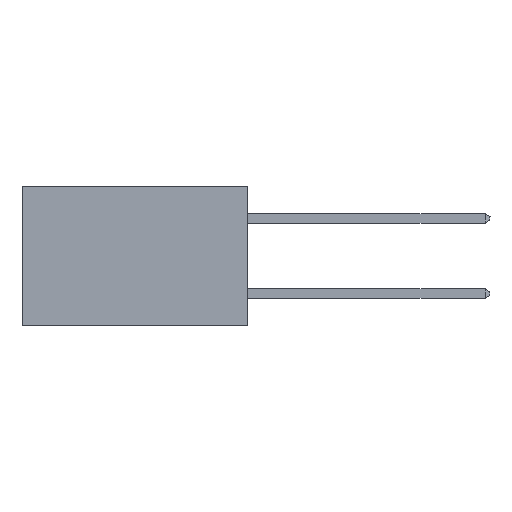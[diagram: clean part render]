
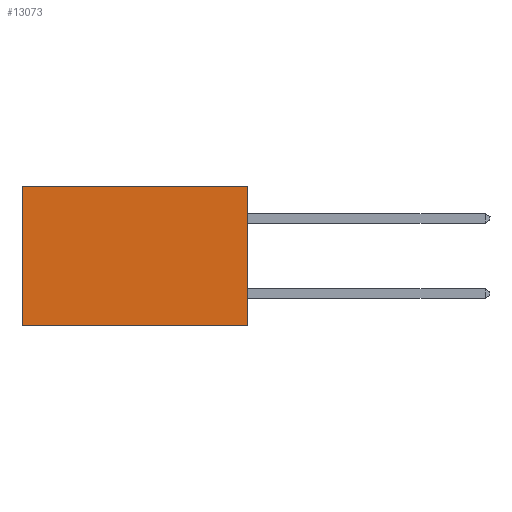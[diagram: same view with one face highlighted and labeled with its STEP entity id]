
A CAD part, left-side view. The second image highlights one B-rep face of the part: STEP entity #13073.
In plain terms, the highlighted planar face has unit normal (-1, 0, 0).
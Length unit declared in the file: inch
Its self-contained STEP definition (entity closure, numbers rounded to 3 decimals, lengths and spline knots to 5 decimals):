
#404 = CARTESIAN_POINT ( 'NONE',  ( 0.2615, 0.6, -0.37 ) ) ;
#422 = CARTESIAN_POINT ( 'NONE',  ( 0.2615, 0.6, 0. ) ) ;
#670 = CARTESIAN_POINT ( 'NONE',  ( 0.2615, 0.6, -0.37 ) ) ;
#1036 = FACE_OUTER_BOUND ( 'NONE', #8009, .T. ) ;
#2550 = VERTEX_POINT ( 'NONE', #13276 ) ;
#3620 = DIRECTION ( 'NONE',  ( 0., 0., -1. ) ) ;
#3653 = VECTOR ( 'NONE', #6985, 39.37008 ) ;
#4082 = VERTEX_POINT ( 'NONE', #670 ) ;
#4571 = ORIENTED_EDGE ( 'NONE', *, *, #7743, .T. ) ;
#4793 = CARTESIAN_POINT ( 'NONE',  ( 0.2615, 0., -0.37 ) ) ;
#4908 = VECTOR ( 'NONE', #5227, 39.37008 ) ;
#5067 = LINE ( 'NONE', #404, #15256 ) ;
#5227 = DIRECTION ( 'NONE',  ( 0., 1., 0. ) ) ;
#5365 = ORIENTED_EDGE ( 'NONE', *, *, #10840, .F. ) ;
#5797 = DIRECTION ( 'NONE',  ( 1., 0., 0. ) ) ;
#5877 = LINE ( 'NONE', #12953, #3653 ) ;
#5997 = VERTEX_POINT ( 'NONE', #15090 ) ;
#6898 = ORIENTED_EDGE ( 'NONE', *, *, #14724, .T. ) ;
#6985 = DIRECTION ( 'NONE',  ( 0., 0., -1. ) ) ;
#7135 = DIRECTION ( 'NONE',  ( 0., 1., 0. ) ) ;
#7436 = VERTEX_POINT ( 'NONE', #422 ) ;
#7646 = VECTOR ( 'NONE', #7135, 39.37008 ) ;
#7743 = EDGE_CURVE ( 'NONE', #5997, #7436, #13624, .T. ) ;
#8009 = EDGE_LOOP ( 'NONE', ( #6898, #5365, #11584, #4571 ) ) ;
#8851 = DIRECTION ( 'NONE',  ( 0., 0., -1. ) ) ;
#10460 = PLANE ( 'NONE',  #13962 ) ;
#10746 = EDGE_CURVE ( 'NONE', #5997, #2550, #5877, .T. ) ;
#10840 = EDGE_CURVE ( 'NONE', #2550, #4082, #14362, .T. ) ;
#11584 = ORIENTED_EDGE ( 'NONE', *, *, #10746, .F. ) ;
#12953 = CARTESIAN_POINT ( 'NONE',  ( 0.2615, 0., -0.37 ) ) ;
#13073 = ADVANCED_FACE ( 'NONE', ( #1036 ), #10460, .F. ) ;
#13187 = CARTESIAN_POINT ( 'NONE',  ( 0.2615, 0., -0.37 ) ) ;
#13276 = CARTESIAN_POINT ( 'NONE',  ( 0.2615, 0., -0.37 ) ) ;
#13624 = LINE ( 'NONE', #14805, #4908 ) ;
#13962 = AXIS2_PLACEMENT_3D ( 'NONE', #4793, #5797, #3620 ) ;
#14362 = LINE ( 'NONE', #13187, #7646 ) ;
#14724 = EDGE_CURVE ( 'NONE', #7436, #4082, #5067, .T. ) ;
#14805 = CARTESIAN_POINT ( 'NONE',  ( 0.2615, 0., 0. ) ) ;
#15090 = CARTESIAN_POINT ( 'NONE',  ( 0.2615, 0., 0. ) ) ;
#15256 = VECTOR ( 'NONE', #8851, 39.37008 ) ;
